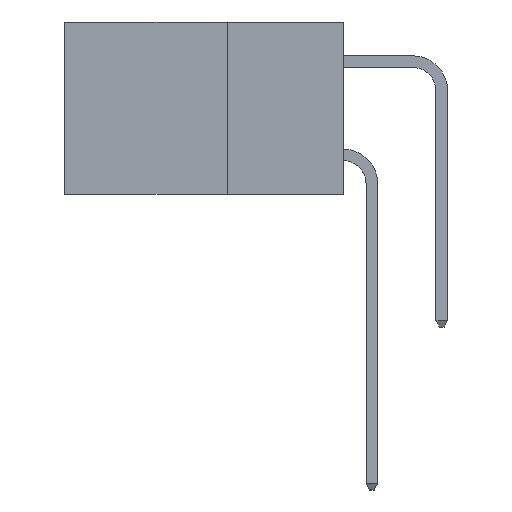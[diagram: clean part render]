
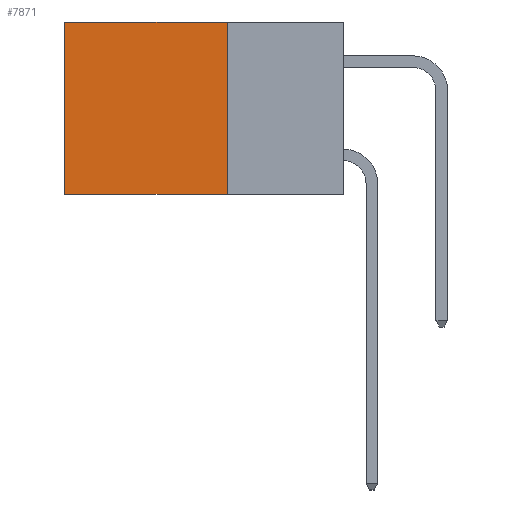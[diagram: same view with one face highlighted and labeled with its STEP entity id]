
A CAD part, left-side view. The second image highlights one B-rep face of the part: STEP entity #7871.
In plain terms, the highlighted planar face has unit normal (-1, 0, 0).
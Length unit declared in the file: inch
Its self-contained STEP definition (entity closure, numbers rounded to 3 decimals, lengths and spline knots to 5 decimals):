
#84 = VECTOR ( 'NONE', #7603, 39.37008 ) ;
#120 = PLANE ( 'NONE',  #11747 ) ;
#357 = LINE ( 'NONE', #7004, #9796 ) ;
#1150 = CARTESIAN_POINT ( 'NONE',  ( 0.2615, 0.6, 0. ) ) ;
#1504 = LINE ( 'NONE', #9648, #4202 ) ;
#1715 = VERTEX_POINT ( 'NONE', #9698 ) ;
#1868 = LINE ( 'NONE', #7385, #8586 ) ;
#2574 = CARTESIAN_POINT ( 'NONE',  ( 0.2615, 0.6, -0.37 ) ) ;
#2813 = DIRECTION ( 'NONE',  ( 0., 0., -1. ) ) ;
#4113 = EDGE_CURVE ( 'NONE', #1715, #9985, #1504, .T. ) ;
#4202 = VECTOR ( 'NONE', #2813, 39.37008 ) ;
#4213 = LINE ( 'NONE', #8417, #84 ) ;
#4240 = FACE_OUTER_BOUND ( 'NONE', #10717, .T. ) ;
#5518 = VERTEX_POINT ( 'NONE', #1150 ) ;
#5806 = ORIENTED_EDGE ( 'NONE', *, *, #11302, .T. ) ;
#6259 = EDGE_CURVE ( 'NONE', #5518, #11823, #1868, .T. ) ;
#6270 = CARTESIAN_POINT ( 'NONE',  ( 0.2615, 0.25, -0.37 ) ) ;
#6452 = CARTESIAN_POINT ( 'NONE',  ( 0.2615, 0.25, -0.37 ) ) ;
#7004 = CARTESIAN_POINT ( 'NONE',  ( 0.2615, 0.25, -0.37 ) ) ;
#7385 = CARTESIAN_POINT ( 'NONE',  ( 0.2615, 0.6, -0.37 ) ) ;
#7603 = DIRECTION ( 'NONE',  ( 0., 1., 0. ) ) ;
#7871 = ADVANCED_FACE ( 'NONE', ( #4240 ), #120, .F. ) ;
#8323 = DIRECTION ( 'NONE',  ( 0., 0., -1. ) ) ;
#8408 = DIRECTION ( 'NONE',  ( 1., 0., 0. ) ) ;
#8417 = CARTESIAN_POINT ( 'NONE',  ( 0.2615, 0.25, 0. ) ) ;
#8586 = VECTOR ( 'NONE', #8323, 39.37008 ) ;
#8841 = DIRECTION ( 'NONE',  ( 0., 1., 0. ) ) ;
#9139 = ORIENTED_EDGE ( 'NONE', *, *, #6259, .T. ) ;
#9298 = DIRECTION ( 'NONE',  ( 0., 0., -1. ) ) ;
#9648 = CARTESIAN_POINT ( 'NONE',  ( 0.2615, 0.25, -0.37 ) ) ;
#9698 = CARTESIAN_POINT ( 'NONE',  ( 0.2615, 0.25, 0. ) ) ;
#9796 = VECTOR ( 'NONE', #8841, 39.37008 ) ;
#9985 = VERTEX_POINT ( 'NONE', #6270 ) ;
#10717 = EDGE_LOOP ( 'NONE', ( #9139, #10851, #11714, #5806 ) ) ;
#10851 = ORIENTED_EDGE ( 'NONE', *, *, #11780, .F. ) ;
#11302 = EDGE_CURVE ( 'NONE', #1715, #5518, #4213, .T. ) ;
#11714 = ORIENTED_EDGE ( 'NONE', *, *, #4113, .F. ) ;
#11747 = AXIS2_PLACEMENT_3D ( 'NONE', #6452, #8408, #9298 ) ;
#11780 = EDGE_CURVE ( 'NONE', #9985, #11823, #357, .T. ) ;
#11823 = VERTEX_POINT ( 'NONE', #2574 ) ;
